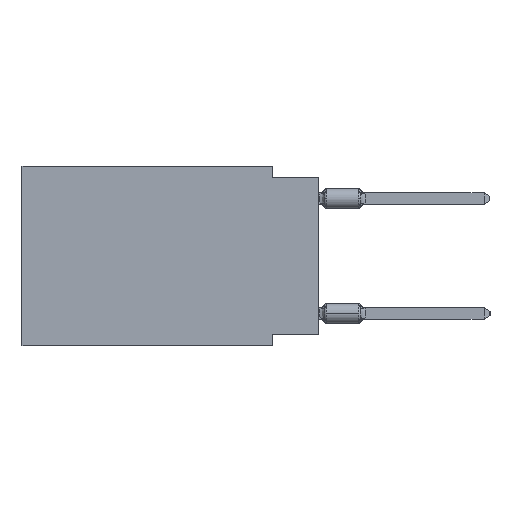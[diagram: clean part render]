
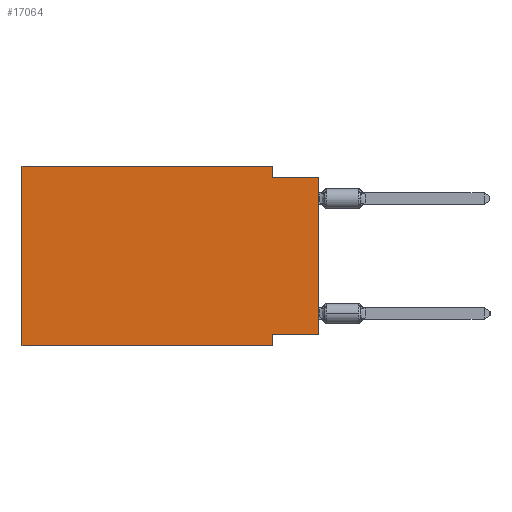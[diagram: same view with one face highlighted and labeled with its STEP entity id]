
A CAD part, left-side view. The second image highlights one B-rep face of the part: STEP entity #17064.
In plain terms, the highlighted planar face has unit normal (-1, 0, 0).
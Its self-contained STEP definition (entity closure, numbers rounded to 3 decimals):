
#1344 = VERTEX_POINT ( 'NONE', #28975 ) ;
#2031 = DIRECTION ( 'NONE',  ( 0., 0., 1. ) ) ;
#2668 = EDGE_CURVE ( 'NONE', #17656, #5982, #29554, .T. ) ;
#2696 = VECTOR ( 'NONE', #16507, 1000. ) ;
#2911 = EDGE_CURVE ( 'NONE', #17656, #1344, #17498, .T. ) ;
#3222 = LINE ( 'NONE', #12381, #10861 ) ;
#3239 = VECTOR ( 'NONE', #2031, 1000. ) ;
#3298 = CARTESIAN_POINT ( 'NONE',  ( 0., 2.54, -9.906 ) ) ;
#3682 = VECTOR ( 'NONE', #25612, 1000. ) ;
#3907 = VECTOR ( 'NONE', #13578, 1000. ) ;
#4217 = VECTOR ( 'NONE', #5407, 1000. ) ;
#4612 = ORIENTED_EDGE ( 'NONE', *, *, #10176, .F. ) ;
#5407 = DIRECTION ( 'NONE',  ( 0., 0., -1. ) ) ;
#5559 = EDGE_CURVE ( 'NONE', #9232, #5982, #25891, .T. ) ;
#5982 = VERTEX_POINT ( 'NONE', #10289 ) ;
#6453 = DIRECTION ( 'NONE',  ( 0., 0., -1. ) ) ;
#6820 = CARTESIAN_POINT ( 'NONE',  ( 0., 16.383, -9.906 ) ) ;
#8358 = ORIENTED_EDGE ( 'NONE', *, *, #5559, .F. ) ;
#9232 = VERTEX_POINT ( 'NONE', #27489 ) ;
#10010 = CARTESIAN_POINT ( 'NONE',  ( 0., 16.383, -9.906 ) ) ;
#10176 = EDGE_CURVE ( 'NONE', #1344, #25892, #11443, .T. ) ;
#10289 = CARTESIAN_POINT ( 'NONE',  ( 0., 2.54, -9.906 ) ) ;
#10861 = VECTOR ( 'NONE', #19480, 1000. ) ;
#11443 = LINE ( 'NONE', #28011, #3682 ) ;
#12105 = EDGE_CURVE ( 'NONE', #25892, #13071, #25242, .T. ) ;
#12381 = CARTESIAN_POINT ( 'NONE',  ( 0., 0., -0.635 ) ) ;
#12704 = ORIENTED_EDGE ( 'NONE', *, *, #20824, .T. ) ;
#13071 = VERTEX_POINT ( 'NONE', #23647 ) ;
#13361 = FACE_OUTER_BOUND ( 'NONE', #23559, .T. ) ;
#13464 = CARTESIAN_POINT ( 'NONE',  ( 0., 0., 0. ) ) ;
#13578 = DIRECTION ( 'NONE',  ( 0., -1., 0. ) ) ;
#13756 = ORIENTED_EDGE ( 'NONE', *, *, #2911, .F. ) ;
#13790 = CARTESIAN_POINT ( 'NONE',  ( 0., 2.54, 0. ) ) ;
#14010 = VECTOR ( 'NONE', #25438, 1000. ) ;
#15270 = ORIENTED_EDGE ( 'NONE', *, *, #25025, .F. ) ;
#15335 = CARTESIAN_POINT ( 'NONE',  ( 0., 16.383, 0. ) ) ;
#15689 = EDGE_CURVE ( 'NONE', #20117, #9232, #20626, .T. ) ;
#16507 = DIRECTION ( 'NONE',  ( 0., 0., -1. ) ) ;
#16847 = AXIS2_PLACEMENT_3D ( 'NONE', #15335, #20169, #6453 ) ;
#17064 = ADVANCED_FACE ( 'NONE', ( #13361 ), #29058, .F. ) ;
#17498 = LINE ( 'NONE', #24432, #24624 ) ;
#17517 = CARTESIAN_POINT ( 'NONE',  ( 0., 0., -0.635 ) ) ;
#17656 = VERTEX_POINT ( 'NONE', #10010 ) ;
#18215 = CARTESIAN_POINT ( 'NONE',  ( 0., 0., -9.271 ) ) ;
#18300 = CARTESIAN_POINT ( 'NONE',  ( 0., 2.54, 0. ) ) ;
#18388 = ORIENTED_EDGE ( 'NONE', *, *, #2668, .T. ) ;
#18862 = ORIENTED_EDGE ( 'NONE', *, *, #12105, .F. ) ;
#19480 = DIRECTION ( 'NONE',  ( 0., -1., 0. ) ) ;
#19756 = DIRECTION ( 'NONE',  ( 0., 0., 1. ) ) ;
#20117 = VERTEX_POINT ( 'NONE', #23606 ) ;
#20169 = DIRECTION ( 'NONE',  ( 1., 0., 0. ) ) ;
#20626 = LINE ( 'NONE', #18215, #14010 ) ;
#20824 = EDGE_CURVE ( 'NONE', #20117, #28400, #24928, .T. ) ;
#23559 = EDGE_LOOP ( 'NONE', ( #12704, #15270, #18862, #4612, #13756, #18388, #8358, #27084 ) ) ;
#23606 = CARTESIAN_POINT ( 'NONE',  ( 0., 0., -9.271 ) ) ;
#23647 = CARTESIAN_POINT ( 'NONE',  ( 0., 2.54, -0.635 ) ) ;
#24432 = CARTESIAN_POINT ( 'NONE',  ( 0., 16.383, 0. ) ) ;
#24624 = VECTOR ( 'NONE', #19756, 1000. ) ;
#24928 = LINE ( 'NONE', #13464, #3239 ) ;
#25025 = EDGE_CURVE ( 'NONE', #13071, #28400, #3222, .T. ) ;
#25242 = LINE ( 'NONE', #13790, #2696 ) ;
#25438 = DIRECTION ( 'NONE',  ( 0., 1., 0. ) ) ;
#25612 = DIRECTION ( 'NONE',  ( 0., -1., 0. ) ) ;
#25891 = LINE ( 'NONE', #3298, #4217 ) ;
#25892 = VERTEX_POINT ( 'NONE', #18300 ) ;
#27084 = ORIENTED_EDGE ( 'NONE', *, *, #15689, .F. ) ;
#27489 = CARTESIAN_POINT ( 'NONE',  ( 0., 2.54, -9.271 ) ) ;
#28011 = CARTESIAN_POINT ( 'NONE',  ( 0., 16.383, 0. ) ) ;
#28400 = VERTEX_POINT ( 'NONE', #17517 ) ;
#28975 = CARTESIAN_POINT ( 'NONE',  ( 0., 16.383, 0. ) ) ;
#29058 = PLANE ( 'NONE',  #16847 ) ;
#29554 = LINE ( 'NONE', #6820, #3907 ) ;
